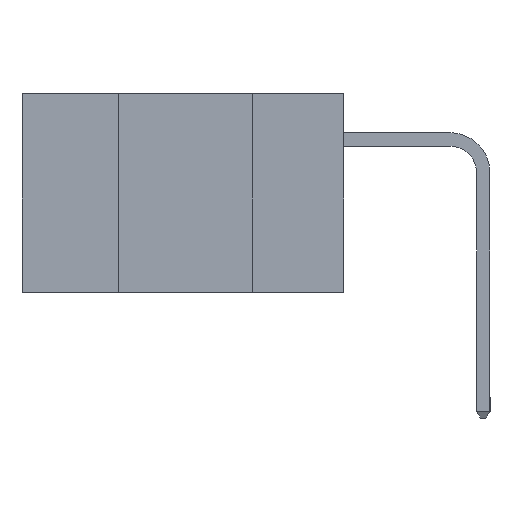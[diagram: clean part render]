
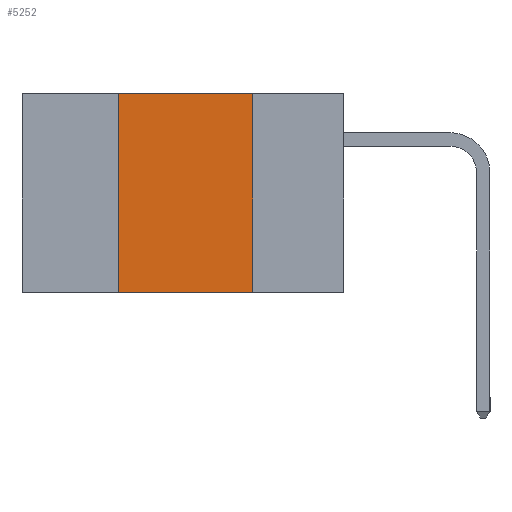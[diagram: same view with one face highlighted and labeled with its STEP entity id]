
A CAD part, left-side view. The second image highlights one B-rep face of the part: STEP entity #5252.
In plain terms, the highlighted planar face has unit normal (-1, 0, 0).
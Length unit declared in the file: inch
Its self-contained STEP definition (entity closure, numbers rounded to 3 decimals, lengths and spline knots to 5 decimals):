
#487 = EDGE_LOOP ( 'NONE', ( #18400, #14994, #11134, #12664 ) ) ;
#716 = EDGE_CURVE ( 'NONE', #14932, #4980, #3616, .T. ) ;
#1278 = VERTEX_POINT ( 'NONE', #17842 ) ;
#1834 = EDGE_CURVE ( 'NONE', #4980, #11938, #11234, .T. ) ;
#2948 = LINE ( 'NONE', #18656, #17907 ) ;
#3616 = LINE ( 'NONE', #4182, #8168 ) ;
#4182 = CARTESIAN_POINT ( 'NONE',  ( 0., 0.6, 0. ) ) ;
#4302 = DIRECTION ( 'NONE',  ( 0., 0., -1. ) ) ;
#4980 = VERTEX_POINT ( 'NONE', #19195 ) ;
#5252 = ADVANCED_FACE ( 'NONE', ( #16536 ), #16777, .F. ) ;
#5523 = CARTESIAN_POINT ( 'NONE',  ( 0., 0.17, -0.37 ) ) ;
#6934 = DIRECTION ( 'NONE',  ( 0., -1., 0. ) ) ;
#7421 = CARTESIAN_POINT ( 'NONE',  ( 0., 0.17, -0.37 ) ) ;
#8168 = VECTOR ( 'NONE', #6934, 39.37008 ) ;
#9160 = EDGE_CURVE ( 'NONE', #1278, #11938, #2948, .T. ) ;
#9728 = DIRECTION ( 'NONE',  ( 0., 0., 1. ) ) ;
#11134 = ORIENTED_EDGE ( 'NONE', *, *, #15793, .F. ) ;
#11234 = LINE ( 'NONE', #7421, #19494 ) ;
#11938 = VERTEX_POINT ( 'NONE', #5523 ) ;
#12664 = ORIENTED_EDGE ( 'NONE', *, *, #9160, .T. ) ;
#14614 = CARTESIAN_POINT ( 'NONE',  ( 0., 0.42, -0.37 ) ) ;
#14932 = VERTEX_POINT ( 'NONE', #17565 ) ;
#14994 = ORIENTED_EDGE ( 'NONE', *, *, #716, .F. ) ;
#15472 = AXIS2_PLACEMENT_3D ( 'NONE', #16661, #16633, #16611 ) ;
#15509 = VECTOR ( 'NONE', #9728, 39.37008 ) ;
#15793 = EDGE_CURVE ( 'NONE', #1278, #14932, #19389, .T. ) ;
#16536 = FACE_OUTER_BOUND ( 'NONE', #487, .T. ) ;
#16611 = DIRECTION ( 'NONE',  ( 0., 0., -1. ) ) ;
#16633 = DIRECTION ( 'NONE',  ( 1., 0., 0. ) ) ;
#16661 = CARTESIAN_POINT ( 'NONE',  ( 0., 0.6, 0. ) ) ;
#16777 = PLANE ( 'NONE',  #15472 ) ;
#17565 = CARTESIAN_POINT ( 'NONE',  ( 0., 0.42, 0. ) ) ;
#17842 = CARTESIAN_POINT ( 'NONE',  ( 0., 0.42, -0.37 ) ) ;
#17907 = VECTOR ( 'NONE', #18626, 39.37008 ) ;
#18400 = ORIENTED_EDGE ( 'NONE', *, *, #1834, .F. ) ;
#18626 = DIRECTION ( 'NONE',  ( 0., -1., 0. ) ) ;
#18656 = CARTESIAN_POINT ( 'NONE',  ( 0., 0.6, -0.37 ) ) ;
#19195 = CARTESIAN_POINT ( 'NONE',  ( 0., 0.17, 0. ) ) ;
#19389 = LINE ( 'NONE', #14614, #15509 ) ;
#19494 = VECTOR ( 'NONE', #4302, 39.37008 ) ;
